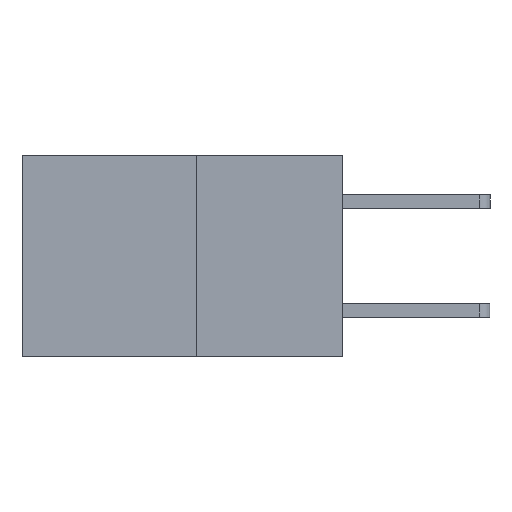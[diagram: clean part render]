
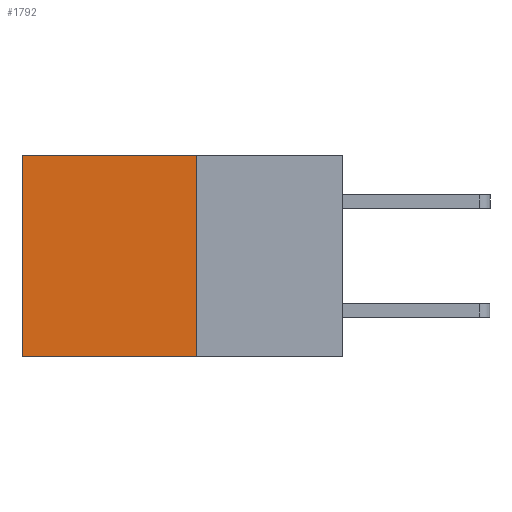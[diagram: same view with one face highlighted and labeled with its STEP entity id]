
A CAD part, left-side view. The second image highlights one B-rep face of the part: STEP entity #1792.
In plain terms, the highlighted planar face has unit normal (-1, 0, 0).
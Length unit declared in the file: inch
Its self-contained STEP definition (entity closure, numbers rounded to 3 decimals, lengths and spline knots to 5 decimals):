
#629 = ORIENTED_EDGE ( 'NONE', *, *, #7982, .T. ) ;
#738 = CARTESIAN_POINT ( 'NONE',  ( 0.277, 0.27, 0. ) ) ;
#1061 = CARTESIAN_POINT ( 'NONE',  ( 0.277, 0.27, -0.37 ) ) ;
#1595 = DIRECTION ( 'NONE',  ( 0., 1., 0. ) ) ;
#1792 = ADVANCED_FACE ( 'NONE', ( #6804 ), #6622, .F. ) ;
#1819 = ORIENTED_EDGE ( 'NONE', *, *, #7627, .F. ) ;
#2044 = VERTEX_POINT ( 'NONE', #4882 ) ;
#2085 = DIRECTION ( 'NONE',  ( 0., 0., -1. ) ) ;
#2233 = DIRECTION ( 'NONE',  ( 0., 0., -1. ) ) ;
#2279 = VERTEX_POINT ( 'NONE', #1061 ) ;
#2420 = CARTESIAN_POINT ( 'NONE',  ( 0.277, 0.59, -0.37 ) ) ;
#2453 = ORIENTED_EDGE ( 'NONE', *, *, #7897, .T. ) ;
#2652 = CARTESIAN_POINT ( 'NONE',  ( 0.277, 0.27, -0.37 ) ) ;
#3259 = DIRECTION ( 'NONE',  ( 0., 1., 0. ) ) ;
#3618 = VECTOR ( 'NONE', #1595, 39.37008 ) ;
#3672 = VERTEX_POINT ( 'NONE', #4075 ) ;
#3901 = LINE ( 'NONE', #6976, #6932 ) ;
#3978 = CARTESIAN_POINT ( 'NONE',  ( 0.277, 0.27, -0.37 ) ) ;
#4075 = CARTESIAN_POINT ( 'NONE',  ( 0.277, 0.27, 0. ) ) ;
#4127 = DIRECTION ( 'NONE',  ( 0., 0., -1. ) ) ;
#4699 = LINE ( 'NONE', #2652, #7607 ) ;
#4882 = CARTESIAN_POINT ( 'NONE',  ( 0.277, 0.59, 0. ) ) ;
#5312 = CARTESIAN_POINT ( 'NONE',  ( 0.277, 0.59, -0.37 ) ) ;
#5427 = VERTEX_POINT ( 'NONE', #2420 ) ;
#5701 = ORIENTED_EDGE ( 'NONE', *, *, #7758, .F. ) ;
#6622 = PLANE ( 'NONE',  #7233 ) ;
#6778 = DIRECTION ( 'NONE',  ( 1., 0., 0. ) ) ;
#6804 = FACE_OUTER_BOUND ( 'NONE', #7503, .T. ) ;
#6821 = LINE ( 'NONE', #738, #3618 ) ;
#6932 = VECTOR ( 'NONE', #2085, 39.37008 ) ;
#6976 = CARTESIAN_POINT ( 'NONE',  ( 0.277, 0.27, -0.37 ) ) ;
#7233 = AXIS2_PLACEMENT_3D ( 'NONE', #3978, #6778, #4127 ) ;
#7341 = VECTOR ( 'NONE', #2233, 39.37008 ) ;
#7503 = EDGE_LOOP ( 'NONE', ( #2453, #1819, #5701, #629 ) ) ;
#7513 = LINE ( 'NONE', #5312, #7341 ) ;
#7607 = VECTOR ( 'NONE', #3259, 39.37008 ) ;
#7627 = EDGE_CURVE ( 'NONE', #2279, #5427, #4699, .T. ) ;
#7758 = EDGE_CURVE ( 'NONE', #3672, #2279, #3901, .T. ) ;
#7897 = EDGE_CURVE ( 'NONE', #2044, #5427, #7513, .T. ) ;
#7982 = EDGE_CURVE ( 'NONE', #3672, #2044, #6821, .T. ) ;
